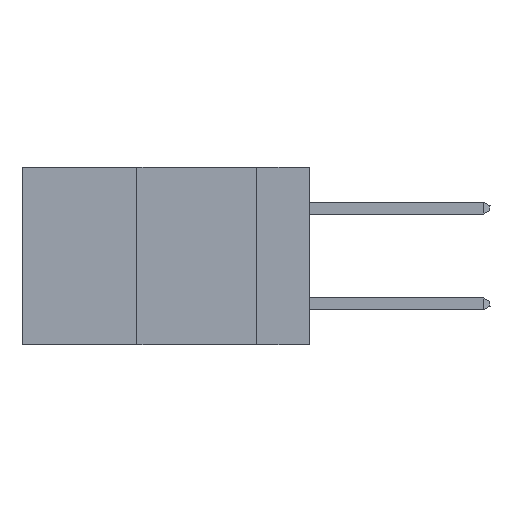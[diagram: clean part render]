
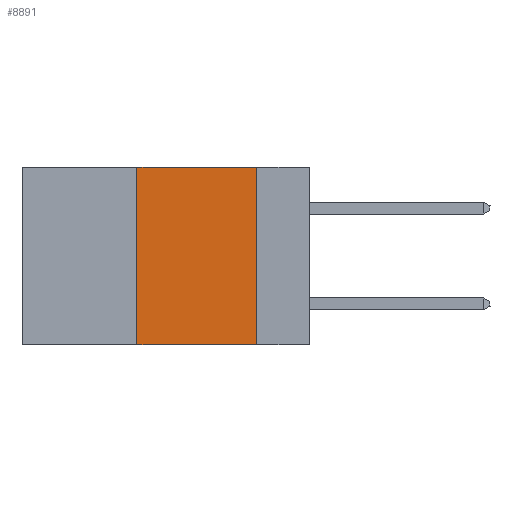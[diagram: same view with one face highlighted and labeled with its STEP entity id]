
A CAD part, left-side view. The second image highlights one B-rep face of the part: STEP entity #8891.
In plain terms, the highlighted planar face has unit normal (-1, 0, 0).
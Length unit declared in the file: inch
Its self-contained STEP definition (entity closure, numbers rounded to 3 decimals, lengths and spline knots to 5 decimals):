
#2778 = DIRECTION ( 'NONE',  ( 0., 0., 1. ) ) ;
#2810 = LINE ( 'NONE', #20451, #4680 ) ;
#3313 = VECTOR ( 'NONE', #12699, 39.37008 ) ;
#4148 = VECTOR ( 'NONE', #15246, 39.37008 ) ;
#4680 = VECTOR ( 'NONE', #2778, 39.37008 ) ;
#5851 = EDGE_CURVE ( 'NONE', #22810, #17578, #10136, .T. ) ;
#6449 = CARTESIAN_POINT ( 'NONE',  ( 0., 0.36, -0.37 ) ) ;
#6540 = LINE ( 'NONE', #32542, #3313 ) ;
#7479 = CARTESIAN_POINT ( 'NONE',  ( 0., 0.11, -0.37 ) ) ;
#7933 = PLANE ( 'NONE',  #19961 ) ;
#8891 = ADVANCED_FACE ( 'NONE', ( #36158 ), #7933, .F. ) ;
#9168 = CARTESIAN_POINT ( 'NONE',  ( 0., 0.6, 0. ) ) ;
#9826 = ORIENTED_EDGE ( 'NONE', *, *, #5851, .F. ) ;
#10136 = LINE ( 'NONE', #9168, #4148 ) ;
#10465 = ORIENTED_EDGE ( 'NONE', *, *, #23067, .F. ) ;
#12545 = EDGE_CURVE ( 'NONE', #18376, #17949, #6540, .T. ) ;
#12699 = DIRECTION ( 'NONE',  ( 0., -1., 0. ) ) ;
#12772 = ORIENTED_EDGE ( 'NONE', *, *, #27142, .F. ) ;
#15246 = DIRECTION ( 'NONE',  ( 0., -1., 0. ) ) ;
#15994 = CARTESIAN_POINT ( 'NONE',  ( 0., 0.11, 0. ) ) ;
#16678 = DIRECTION ( 'NONE',  ( 0., 0., -1. ) ) ;
#17578 = VERTEX_POINT ( 'NONE', #23633 ) ;
#17949 = VERTEX_POINT ( 'NONE', #7479 ) ;
#18376 = VERTEX_POINT ( 'NONE', #6449 ) ;
#19961 = AXIS2_PLACEMENT_3D ( 'NONE', #34326, #25397, #16678 ) ;
#20451 = CARTESIAN_POINT ( 'NONE',  ( 0., 0.36, 0. ) ) ;
#21047 = CARTESIAN_POINT ( 'NONE',  ( 0., 0.36, 0. ) ) ;
#22810 = VERTEX_POINT ( 'NONE', #21047 ) ;
#22815 = EDGE_LOOP ( 'NONE', ( #10465, #9826, #12772, #29528 ) ) ;
#23067 = EDGE_CURVE ( 'NONE', #17578, #17949, #27399, .T. ) ;
#23260 = VECTOR ( 'NONE', #34149, 39.37008 ) ;
#23633 = CARTESIAN_POINT ( 'NONE',  ( 0., 0.11, 0. ) ) ;
#25397 = DIRECTION ( 'NONE',  ( 1., 0., 0. ) ) ;
#27142 = EDGE_CURVE ( 'NONE', #18376, #22810, #2810, .T. ) ;
#27399 = LINE ( 'NONE', #15994, #23260 ) ;
#29528 = ORIENTED_EDGE ( 'NONE', *, *, #12545, .T. ) ;
#32542 = CARTESIAN_POINT ( 'NONE',  ( 0., 0.6, -0.37 ) ) ;
#34149 = DIRECTION ( 'NONE',  ( 0., 0., -1. ) ) ;
#34326 = CARTESIAN_POINT ( 'NONE',  ( 0., 0.6, 0. ) ) ;
#36158 = FACE_OUTER_BOUND ( 'NONE', #22815, .T. ) ;
